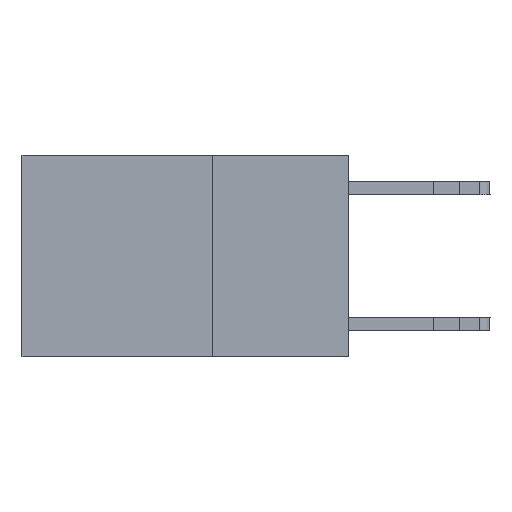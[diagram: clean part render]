
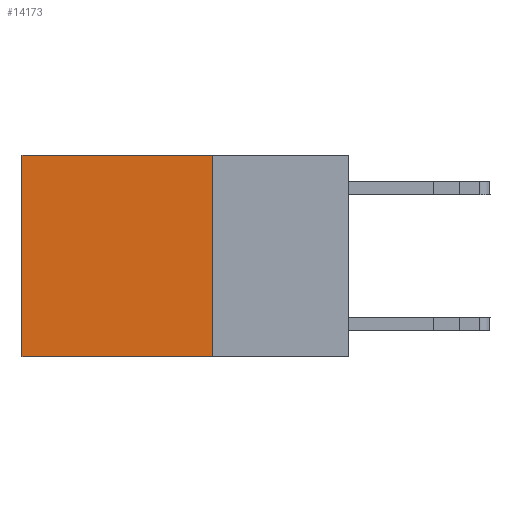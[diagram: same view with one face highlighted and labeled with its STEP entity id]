
A CAD part, left-side view. The second image highlights one B-rep face of the part: STEP entity #14173.
In plain terms, the highlighted planar face has unit normal (-1, 0, 0).
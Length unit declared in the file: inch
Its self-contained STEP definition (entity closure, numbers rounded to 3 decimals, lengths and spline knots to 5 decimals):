
#62 = CARTESIAN_POINT ( 'NONE',  ( 0.2625, 0.25, 0. ) ) ;
#78 = DIRECTION ( 'NONE',  ( 0., 0., -1. ) ) ;
#282 = VERTEX_POINT ( 'NONE', #12119 ) ;
#362 = LINE ( 'NONE', #2752, #7645 ) ;
#518 = DIRECTION ( 'NONE',  ( 0., 1., 0. ) ) ;
#758 = CARTESIAN_POINT ( 'NONE',  ( 0.2625, 0.25, 0. ) ) ;
#764 = ORIENTED_EDGE ( 'NONE', *, *, #9435, .T. ) ;
#886 = VECTOR ( 'NONE', #78, 39.37008 ) ;
#2160 = VECTOR ( 'NONE', #12676, 39.37008 ) ;
#2579 = VECTOR ( 'NONE', #12080, 39.37008 ) ;
#2614 = CARTESIAN_POINT ( 'NONE',  ( 0.2625, 0.25, 0. ) ) ;
#2710 = AXIS2_PLACEMENT_3D ( 'NONE', #3127, #14615, #3053 ) ;
#2752 = CARTESIAN_POINT ( 'NONE',  ( 0.2625, 0.25, -0.37 ) ) ;
#2902 = ORIENTED_EDGE ( 'NONE', *, *, #6092, .T. ) ;
#3053 = DIRECTION ( 'NONE',  ( 0., 0., -1. ) ) ;
#3127 = CARTESIAN_POINT ( 'NONE',  ( 0.2625, 0.25, 0. ) ) ;
#3819 = LINE ( 'NONE', #2614, #2160 ) ;
#3894 = CARTESIAN_POINT ( 'NONE',  ( 0.2625, 0.6, 0. ) ) ;
#4554 = EDGE_CURVE ( 'NONE', #12556, #13813, #13550, .T. ) ;
#4623 = ORIENTED_EDGE ( 'NONE', *, *, #6616, .F. ) ;
#5452 = PLANE ( 'NONE',  #2710 ) ;
#5779 = CARTESIAN_POINT ( 'NONE',  ( 0.2625, 0.25, -0.37 ) ) ;
#6092 = EDGE_CURVE ( 'NONE', #14066, #282, #11091, .T. ) ;
#6616 = EDGE_CURVE ( 'NONE', #13813, #282, #362, .T. ) ;
#7645 = VECTOR ( 'NONE', #518, 39.37008 ) ;
#9232 = CARTESIAN_POINT ( 'NONE',  ( 0.2625, 0.6, 0. ) ) ;
#9435 = EDGE_CURVE ( 'NONE', #12556, #14066, #3819, .T. ) ;
#11091 = LINE ( 'NONE', #9232, #886 ) ;
#12069 = ORIENTED_EDGE ( 'NONE', *, *, #4554, .F. ) ;
#12080 = DIRECTION ( 'NONE',  ( 0., 0., -1. ) ) ;
#12119 = CARTESIAN_POINT ( 'NONE',  ( 0.2625, 0.6, -0.37 ) ) ;
#12347 = FACE_OUTER_BOUND ( 'NONE', #12796, .T. ) ;
#12556 = VERTEX_POINT ( 'NONE', #62 ) ;
#12676 = DIRECTION ( 'NONE',  ( 0., 1., 0. ) ) ;
#12796 = EDGE_LOOP ( 'NONE', ( #2902, #4623, #12069, #764 ) ) ;
#13550 = LINE ( 'NONE', #758, #2579 ) ;
#13813 = VERTEX_POINT ( 'NONE', #5779 ) ;
#14066 = VERTEX_POINT ( 'NONE', #3894 ) ;
#14173 = ADVANCED_FACE ( 'NONE', ( #12347 ), #5452, .F. ) ;
#14615 = DIRECTION ( 'NONE',  ( 1., 0., 0. ) ) ;
